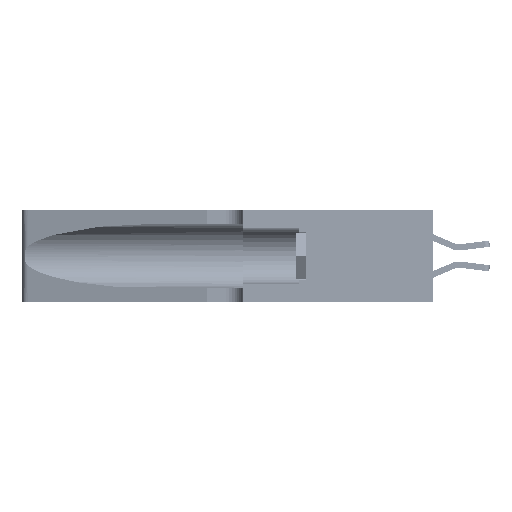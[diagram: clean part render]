
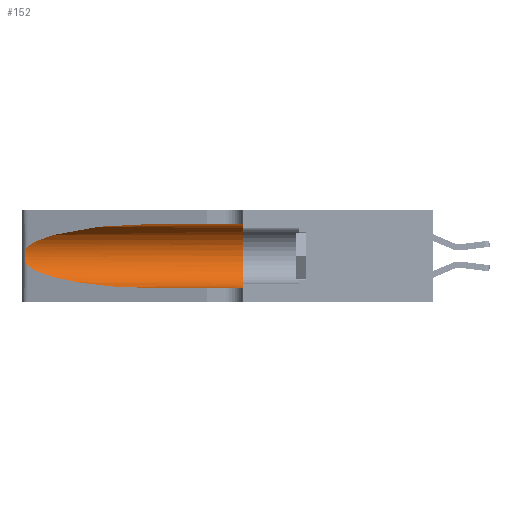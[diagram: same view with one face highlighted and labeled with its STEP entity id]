
A CAD part, left-side view. The second image highlights one B-rep face of the part: STEP entity #152.
In plain terms, the highlighted cylindrical face has radius 3.308 mm (diameter 6.617 mm), a partial arc.
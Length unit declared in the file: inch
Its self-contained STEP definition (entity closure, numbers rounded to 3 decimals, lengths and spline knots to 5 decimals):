
#152 = ADVANCED_FACE ( 'NONE', ( #8167 ), #20239, .F. ) ;
#298 = VERTEX_POINT ( 'NONE', #26270 ) ;
#300 = VERTEX_POINT ( 'NONE', #19686 ) ;
#1037 = CARTESIAN_POINT ( 'NONE',  ( 0.1305, 0.72297, 0.05475 ) ) ;
#1296 = CARTESIAN_POINT ( 'NONE',  ( 0.25487, 1.22718, 0.22369 ) ) ;
#1652 = DIRECTION ( 'NONE',  ( 0., 0., 1. ) ) ;
#1986 = EDGE_CURVE ( 'NONE', #11354, #300, #14075, .T. ) ;
#2442 =( BOUNDED_CURVE ( )  B_SPLINE_CURVE ( 3, ( #4205, #13816, #17174, #1037 ),
 .UNSPECIFIED., .F., .F. ) 
 B_SPLINE_CURVE_WITH_KNOTS ( ( 4, 4 ),
 ( 3.44316, 4.71239 ),
 .UNSPECIFIED. ) 
 CURVE ( )  GEOMETRIC_REPRESENTATION_ITEM ( )  RATIONAL_B_SPLINE_CURVE ( ( 1., 0.87, 0.87, 1. ) ) 
 REPRESENTATION_ITEM ( '' )  );
#2718 = EDGE_CURVE ( 'NONE', #298, #39864, #6276, .T. ) ;
#2721 = DIRECTION ( 'NONE',  ( 0., -1., 0. ) ) ;
#3362 = EDGE_CURVE ( 'NONE', #29885, #300, #3896, .T. ) ;
#3747 = CARTESIAN_POINT ( 'NONE',  ( 0.25487, 1.22718, 0.14631 ) ) ;
#3896 = LINE ( 'NONE', #12284, #33568 ) ;
#4205 = CARTESIAN_POINT ( 'NONE',  ( 0.25487, 1.22718, 0.14631 ) ) ;
#4956 = CARTESIAN_POINT ( 'NONE',  ( 0.1305, 0.35, 0.185 ) ) ;
#5979 = CARTESIAN_POINT ( 'NONE',  ( 0.25639, 1.23184, 0.21858 ) ) ;
#6276 = B_SPLINE_CURVE_WITH_KNOTS ( 'NONE', 3,
 ( #1296, #8357, #5979, #9980, #19393, #25713, #29051, #13111, #39355, #17761, #17823, #40451, #20386, #3747 ),
 .UNSPECIFIED., .F., .F.,
 ( 4, 2, 2, 2, 2, 2, 4 ),
 ( 0., 0.00027, 0.00053, 0.00107, 0.0016, 0.00187, 0.00214 ),
 .UNSPECIFIED. ) ;
#6361 = DIRECTION ( 'NONE',  ( 0., 0., -1. ) ) ;
#6985 = CARTESIAN_POINT ( 'NONE',  ( 0.25487, 1.22718, 0.22369 ) ) ;
#7245 = CARTESIAN_POINT ( 'NONE',  ( 0.1305, 0.35, 0.31525 ) ) ;
#8167 = FACE_OUTER_BOUND ( 'NONE', #8439, .T. ) ;
#8357 = CARTESIAN_POINT ( 'NONE',  ( 0.25555, 1.22994, 0.2215 ) ) ;
#8439 = EDGE_LOOP ( 'NONE', ( #41294, #23874, #39635, #9741, #9421, #15651 ) ) ;
#9302 = DIRECTION ( 'NONE',  ( 0., -1., 0. ) ) ;
#9421 = ORIENTED_EDGE ( 'NONE', *, *, #1986, .F. ) ;
#9741 = ORIENTED_EDGE ( 'NONE', *, *, #3362, .T. ) ;
#9980 = CARTESIAN_POINT ( 'NONE',  ( 0.25787, 1.23484, 0.2124 ) ) ;
#11354 = VERTEX_POINT ( 'NONE', #7245 ) ;
#12284 = CARTESIAN_POINT ( 'NONE',  ( 0.1305, 1.61858, 0.05475 ) ) ;
#13111 = CARTESIAN_POINT ( 'NONE',  ( 0.26075, 1.23896, 0.178 ) ) ;
#13816 = CARTESIAN_POINT ( 'NONE',  ( 0.2373, 1.15595, 0.08982 ) ) ;
#14075 = CIRCLE ( 'NONE', #17399, 0.13025 ) ;
#15143 = CARTESIAN_POINT ( 'NONE',  ( 0.25487, 1.22718, 0.14631 ) ) ;
#15525 = CARTESIAN_POINT ( 'NONE',  ( 0.1305, 1.61858, 0.185 ) ) ;
#15651 = ORIENTED_EDGE ( 'NONE', *, *, #38713, .F. ) ;
#15915 = CARTESIAN_POINT ( 'NONE',  ( 0.1305, 0.72297, 0.05475 ) ) ;
#17174 = CARTESIAN_POINT ( 'NONE',  ( 0.18966, 0.96281, 0.05475 ) ) ;
#17399 = AXIS2_PLACEMENT_3D ( 'NONE', #4956, #36655, #1652 ) ;
#17761 = CARTESIAN_POINT ( 'NONE',  ( 0.25856, 1.23593, 0.16098 ) ) ;
#17823 = CARTESIAN_POINT ( 'NONE',  ( 0.25789, 1.23486, 0.15765 ) ) ;
#19270 = CARTESIAN_POINT ( 'NONE',  ( 0.1305, 1.61858, 0.31525 ) ) ;
#19393 = CARTESIAN_POINT ( 'NONE',  ( 0.25854, 1.2359, 0.20912 ) ) ;
#19686 = CARTESIAN_POINT ( 'NONE',  ( 0.1305, 0.35, 0.05475 ) ) ;
#20239 = CYLINDRICAL_SURFACE ( 'NONE', #34255, 0.13025 ) ;
#20386 = CARTESIAN_POINT ( 'NONE',  ( 0.25555, 1.22993, 0.14849 ) ) ;
#23272 = VERTEX_POINT ( 'NONE', #40854 ) ;
#23874 = ORIENTED_EDGE ( 'NONE', *, *, #2718, .T. ) ;
#25713 = CARTESIAN_POINT ( 'NONE',  ( 0.26018, 1.23835, 0.19895 ) ) ;
#26270 = CARTESIAN_POINT ( 'NONE',  ( 0.25487, 1.22718, 0.22369 ) ) ;
#29051 = CARTESIAN_POINT ( 'NONE',  ( 0.26075, 1.23896, 0.19203 ) ) ;
#29885 = VERTEX_POINT ( 'NONE', #15915 ) ;
#30144 = EDGE_CURVE ( 'NONE', #39864, #29885, #2442, .T. ) ;
#32666 = EDGE_CURVE ( 'NONE', #23272, #298, #38090, .T. ) ;
#32963 = CARTESIAN_POINT ( 'NONE',  ( 0.2373, 1.15595, 0.28018 ) ) ;
#33568 = VECTOR ( 'NONE', #9302, 39.37008 ) ;
#34255 = AXIS2_PLACEMENT_3D ( 'NONE', #15525, #2721, #6361 ) ;
#34957 = DIRECTION ( 'NONE',  ( 0., -1., 0. ) ) ;
#35827 = LINE ( 'NONE', #19270, #36334 ) ;
#35869 = CARTESIAN_POINT ( 'NONE',  ( 0.18966, 0.96281, 0.31525 ) ) ;
#36334 = VECTOR ( 'NONE', #34957, 39.37008 ) ;
#36655 = DIRECTION ( 'NONE',  ( 0., 1., 0. ) ) ;
#38090 =( BOUNDED_CURVE ( )  B_SPLINE_CURVE ( 3, ( #38893, #35869, #32963, #6985 ),
 .UNSPECIFIED., .F., .F. ) 
 B_SPLINE_CURVE_WITH_KNOTS ( ( 4, 4 ),
 ( 1.5708, 2.84003 ),
 .UNSPECIFIED. ) 
 CURVE ( )  GEOMETRIC_REPRESENTATION_ITEM ( )  RATIONAL_B_SPLINE_CURVE ( ( 1., 0.87, 0.87, 1. ) ) 
 REPRESENTATION_ITEM ( '' )  );
#38713 = EDGE_CURVE ( 'NONE', #23272, #11354, #35827, .T. ) ;
#38893 = CARTESIAN_POINT ( 'NONE',  ( 0.1305, 0.72297, 0.31525 ) ) ;
#39355 = CARTESIAN_POINT ( 'NONE',  ( 0.26017, 1.23833, 0.17102 ) ) ;
#39635 = ORIENTED_EDGE ( 'NONE', *, *, #30144, .T. ) ;
#39864 = VERTEX_POINT ( 'NONE', #15143 ) ;
#40451 = CARTESIAN_POINT ( 'NONE',  ( 0.25639, 1.23186, 0.15144 ) ) ;
#40854 = CARTESIAN_POINT ( 'NONE',  ( 0.1305, 0.72297, 0.31525 ) ) ;
#41294 = ORIENTED_EDGE ( 'NONE', *, *, #32666, .T. ) ;
